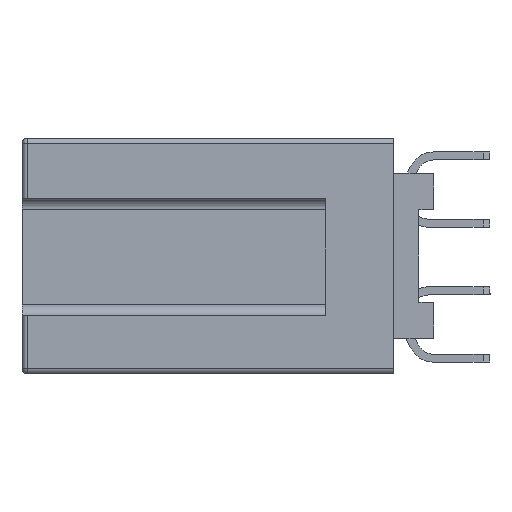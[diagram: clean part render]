
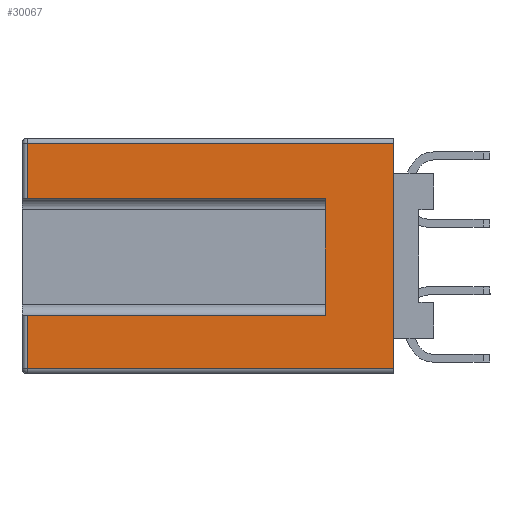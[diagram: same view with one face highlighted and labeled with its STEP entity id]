
A CAD part, left-side view. The second image highlights one B-rep face of the part: STEP entity #30067.
In plain terms, the highlighted planar face has unit normal (-1, 0, 0).
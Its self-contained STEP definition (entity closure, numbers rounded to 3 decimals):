
#11 = VERTEX_POINT ( 'NONE', #42327 ) ;
#124 = LINE ( 'NONE', #44586, #46737 ) ;
#1131 = CARTESIAN_POINT ( 'NONE',  ( 0., 4.07, -2.28 ) ) ;
#2032 = DIRECTION ( 'NONE',  ( 0., 0., -1. ) ) ;
#2430 = DIRECTION ( 'NONE',  ( 0., 1., 0. ) ) ;
#2723 = ORIENTED_EDGE ( 'NONE', *, *, #33493, .T. ) ;
#2844 = ORIENTED_EDGE ( 'NONE', *, *, #13761, .T. ) ;
#3913 = LINE ( 'NONE', #4388, #30658 ) ;
#4016 = VECTOR ( 'NONE', #31944, 1000. ) ;
#4388 = CARTESIAN_POINT ( 'NONE',  ( 0., 15.3, 0. ) ) ;
#4484 = VERTEX_POINT ( 'NONE', #15207 ) ;
#7397 = EDGE_CURVE ( 'NONE', #23891, #25948, #124, .T. ) ;
#9479 = CARTESIAN_POINT ( 'NONE',  ( 0., 15.5, -8.68 ) ) ;
#10237 = CARTESIAN_POINT ( 'NONE',  ( 0., 4.07, -2.28 ) ) ;
#10361 = DIRECTION ( 'NONE',  ( 0., -1., 0. ) ) ;
#10598 = DIRECTION ( 'NONE',  ( 1., 0., 0. ) ) ;
#10749 = EDGE_CURVE ( 'NONE', #45726, #33774, #3913, .T. ) ;
#10916 = DIRECTION ( 'NONE',  ( 0., 0., -1. ) ) ;
#11219 = CARTESIAN_POINT ( 'NONE',  ( 0., 4.07, -2.28 ) ) ;
#13348 = VECTOR ( 'NONE', #47112, 1000. ) ;
#13501 = DIRECTION ( 'NONE',  ( 0., 0., -1. ) ) ;
#13761 = EDGE_CURVE ( 'NONE', #11, #42920, #23949, .T. ) ;
#14587 = LINE ( 'NONE', #29272, #4016 ) ;
#14735 = VECTOR ( 'NONE', #2430, 1000. ) ;
#15207 = CARTESIAN_POINT ( 'NONE',  ( 0., 4.07, -6.68 ) ) ;
#15801 = DIRECTION ( 'NONE',  ( 0., -1., 0. ) ) ;
#15952 = VERTEX_POINT ( 'NONE', #10237 ) ;
#17151 = ORIENTED_EDGE ( 'NONE', *, *, #32219, .T. ) ;
#17725 = CARTESIAN_POINT ( 'NONE',  ( 0., 15.3, -2.28 ) ) ;
#19243 = EDGE_CURVE ( 'NONE', #33774, #25948, #20307, .T. ) ;
#20307 = LINE ( 'NONE', #9479, #26346 ) ;
#20618 = VECTOR ( 'NONE', #2032, 1000. ) ;
#23048 = VECTOR ( 'NONE', #15801, 1000. ) ;
#23891 = VERTEX_POINT ( 'NONE', #27000 ) ;
#23949 = LINE ( 'NONE', #38667, #20618 ) ;
#24969 = LINE ( 'NONE', #11219, #13348 ) ;
#25948 = VERTEX_POINT ( 'NONE', #30493 ) ;
#26093 = EDGE_CURVE ( 'NONE', #42920, #15952, #34119, .T. ) ;
#26346 = VECTOR ( 'NONE', #10361, 1000. ) ;
#26770 = PLANE ( 'NONE',  #39409 ) ;
#27000 = CARTESIAN_POINT ( 'NONE',  ( 0., 1.5, -0.2 ) ) ;
#27719 = ORIENTED_EDGE ( 'NONE', *, *, #7397, .F. ) ;
#27750 = ORIENTED_EDGE ( 'NONE', *, *, #26093, .T. ) ;
#27956 = CARTESIAN_POINT ( 'NONE',  ( 0., 15.3, -6.68 ) ) ;
#29272 = CARTESIAN_POINT ( 'NONE',  ( 0., 15.5, -0.2 ) ) ;
#30067 = ADVANCED_FACE ( 'NONE', ( #30390 ), #26770, .F. ) ;
#30390 = FACE_OUTER_BOUND ( 'NONE', #39422, .T. ) ;
#30493 = CARTESIAN_POINT ( 'NONE',  ( 0., 1.5, -8.68 ) ) ;
#30658 = VECTOR ( 'NONE', #10916, 1000. ) ;
#31543 = EDGE_CURVE ( 'NONE', #4484, #45726, #32759, .T. ) ;
#31944 = DIRECTION ( 'NONE',  ( 0., 1., 0. ) ) ;
#32219 = EDGE_CURVE ( 'NONE', #23891, #11, #14587, .T. ) ;
#32759 = LINE ( 'NONE', #35675, #14735 ) ;
#33493 = EDGE_CURVE ( 'NONE', #15952, #4484, #24969, .T. ) ;
#33576 = DIRECTION ( 'NONE',  ( 0., 0., -1. ) ) ;
#33774 = VERTEX_POINT ( 'NONE', #42731 ) ;
#34119 = LINE ( 'NONE', #1131, #23048 ) ;
#35675 = CARTESIAN_POINT ( 'NONE',  ( 0., 4.07, -6.68 ) ) ;
#37984 = ORIENTED_EDGE ( 'NONE', *, *, #19243, .T. ) ;
#38667 = CARTESIAN_POINT ( 'NONE',  ( 0., 15.3, 0. ) ) ;
#39409 = AXIS2_PLACEMENT_3D ( 'NONE', #41467, #10598, #13501 ) ;
#39422 = EDGE_LOOP ( 'NONE', ( #47233, #37984, #27719, #17151, #2844, #27750, #2723, #40518 ) ) ;
#40518 = ORIENTED_EDGE ( 'NONE', *, *, #31543, .T. ) ;
#41467 = CARTESIAN_POINT ( 'NONE',  ( 0., 15.5, 0. ) ) ;
#42327 = CARTESIAN_POINT ( 'NONE',  ( 0., 15.3, -0.2 ) ) ;
#42731 = CARTESIAN_POINT ( 'NONE',  ( 0., 15.3, -8.68 ) ) ;
#42920 = VERTEX_POINT ( 'NONE', #17725 ) ;
#44586 = CARTESIAN_POINT ( 'NONE',  ( 0., 1.5, 0. ) ) ;
#45726 = VERTEX_POINT ( 'NONE', #27956 ) ;
#46737 = VECTOR ( 'NONE', #33576, 1000. ) ;
#47112 = DIRECTION ( 'NONE',  ( 0., 0., -1. ) ) ;
#47233 = ORIENTED_EDGE ( 'NONE', *, *, #10749, .T. ) ;
